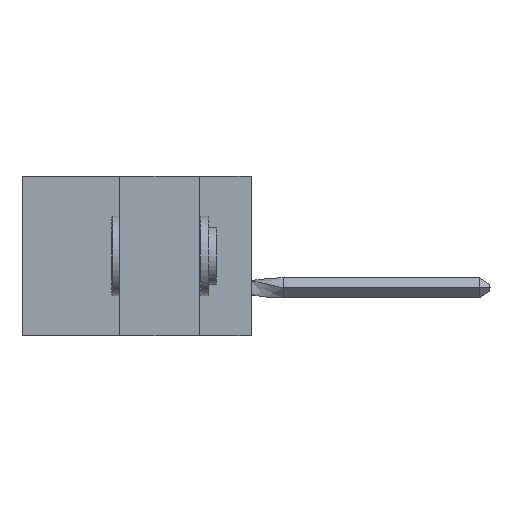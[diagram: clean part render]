
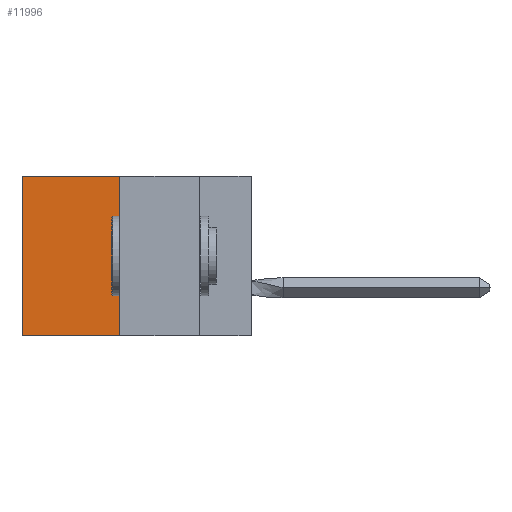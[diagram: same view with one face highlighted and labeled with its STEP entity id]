
A CAD part, left-side view. The second image highlights one B-rep face of the part: STEP entity #11996.
In plain terms, the highlighted planar face has unit normal (-1, 0, 0).
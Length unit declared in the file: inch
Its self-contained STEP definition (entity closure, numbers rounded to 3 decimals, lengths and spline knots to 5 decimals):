
#1058 = ORIENTED_EDGE ( 'NONE', *, *, #7403, .T. ) ;
#1374 = DIRECTION ( 'NONE',  ( 0., 0., -1. ) ) ;
#1563 = VERTEX_POINT ( 'NONE', #13830 ) ;
#2113 = DIRECTION ( 'NONE',  ( 0., 0., -1. ) ) ;
#2857 = EDGE_CURVE ( 'NONE', #11027, #1563, #8141, .T. ) ;
#3115 = VECTOR ( 'NONE', #2113, 39.37008 ) ;
#3537 = CARTESIAN_POINT ( 'NONE',  ( 0.305, 0.413, 0. ) ) ;
#3595 = LINE ( 'NONE', #8065, #3115 ) ;
#4376 = CARTESIAN_POINT ( 'NONE',  ( 0.305, 0.413, 0. ) ) ;
#5212 = VERTEX_POINT ( 'NONE', #14783 ) ;
#5222 = CARTESIAN_POINT ( 'NONE',  ( 0.305, 0.413, -0.5 ) ) ;
#5442 = LINE ( 'NONE', #4376, #13486 ) ;
#5678 = CARTESIAN_POINT ( 'NONE',  ( 0.305, 0.413, -0.5 ) ) ;
#5851 = VERTEX_POINT ( 'NONE', #3537 ) ;
#6857 = CARTESIAN_POINT ( 'NONE',  ( 0.305, 0.413, -0.5 ) ) ;
#7390 = LINE ( 'NONE', #5222, #12107 ) ;
#7403 = EDGE_CURVE ( 'NONE', #5212, #1563, #3595, .T. ) ;
#8065 = CARTESIAN_POINT ( 'NONE',  ( 0.305, 0.72, -0.5 ) ) ;
#8141 = LINE ( 'NONE', #9006, #11661 ) ;
#8447 = EDGE_CURVE ( 'NONE', #5851, #5212, #5442, .T. ) ;
#9006 = CARTESIAN_POINT ( 'NONE',  ( 0.305, 0.413, -0.5 ) ) ;
#9064 = DIRECTION ( 'NONE',  ( 0., 1., 0. ) ) ;
#9453 = AXIS2_PLACEMENT_3D ( 'NONE', #5678, #14946, #1374 ) ;
#11027 = VERTEX_POINT ( 'NONE', #6857 ) ;
#11645 = PLANE ( 'NONE',  #9453 ) ;
#11661 = VECTOR ( 'NONE', #9064, 39.37008 ) ;
#11996 = ADVANCED_FACE ( 'NONE', ( #19364 ), #11645, .F. ) ;
#12107 = VECTOR ( 'NONE', #12613, 39.37008 ) ;
#12613 = DIRECTION ( 'NONE',  ( 0., 0., -1. ) ) ;
#13486 = VECTOR ( 'NONE', #19331, 39.37008 ) ;
#13830 = CARTESIAN_POINT ( 'NONE',  ( 0.305, 0.72, -0.5 ) ) ;
#14602 = EDGE_CURVE ( 'NONE', #5851, #11027, #7390, .T. ) ;
#14691 = ORIENTED_EDGE ( 'NONE', *, *, #2857, .F. ) ;
#14783 = CARTESIAN_POINT ( 'NONE',  ( 0.305, 0.72, 0. ) ) ;
#14946 = DIRECTION ( 'NONE',  ( 1., 0., 0. ) ) ;
#15346 = EDGE_LOOP ( 'NONE', ( #1058, #14691, #16889, #15554 ) ) ;
#15554 = ORIENTED_EDGE ( 'NONE', *, *, #8447, .T. ) ;
#16889 = ORIENTED_EDGE ( 'NONE', *, *, #14602, .F. ) ;
#19331 = DIRECTION ( 'NONE',  ( 0., 1., 0. ) ) ;
#19364 = FACE_OUTER_BOUND ( 'NONE', #15346, .T. ) ;
